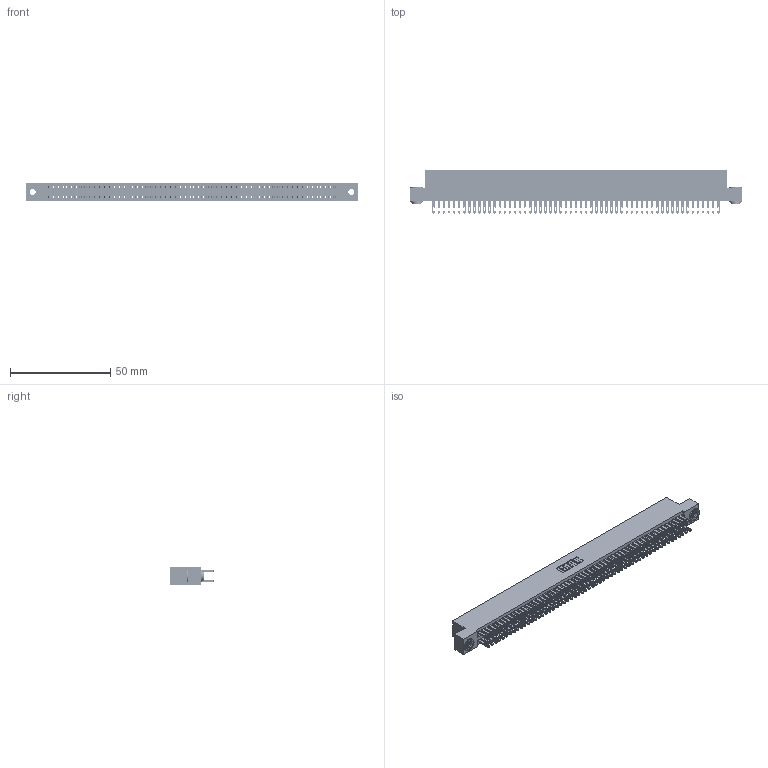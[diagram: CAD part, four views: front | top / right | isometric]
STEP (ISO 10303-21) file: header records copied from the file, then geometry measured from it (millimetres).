
FILE_DESCRIPTION (( 'STEP AP203' ), '1' );
FILE_NAME ('895-114-500-203.STEP', '2020-10-13T13:47:34', ( '' ), ( '' ), 'SwSTEP 2.0', 'SolidWorks 2020', '' );
FILE_SCHEMA (( 'CONFIG_CONTROL_DESIGN' ));
Length unit declared in the file: inch
Products named in the file (4): 345-292-001_345-293-100; 895-114-500-203; 845 Part_Flush Mounting Lugs - 0.156 Dia-TH; 345-250-002_345-250-002-102
Assembly tree (117 placements, depth 2):
  895-114-500-203
    845 Part_Flush Mounting Lugs - 0.156 Dia-TH
    345-292-001_345-293-100  x114
    345-250-002_345-250-002-102  x2
Bounding box: 165.99 x 21.51 x 9.4 mm (x, y, z)
Volume: 16631.3 mm3; surface area: 26242 mm2
Topology: 117 solids, 117 shells, 5408 faces, 16491 edges, 10990 vertices
Faces by surface type: plane 3168, cylinder 2232, cone 8
Entity records: 43284 total; most frequent: CARTESIAN_POINT 7215, ORIENTED_EDGE 7142, DIRECTION 6377, EDGE_CURVE 3571, LINE 3183, VECTOR 3183, VERTEX_POINT 2378, AXIS2_PLACEMENT_3D 1597
